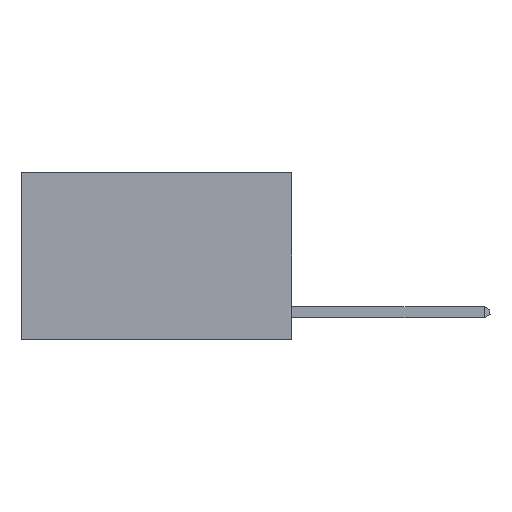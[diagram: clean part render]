
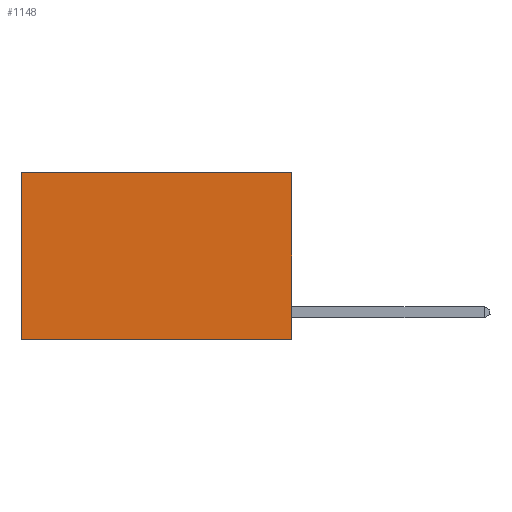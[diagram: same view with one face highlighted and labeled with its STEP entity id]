
A CAD part, left-side view. The second image highlights one B-rep face of the part: STEP entity #1148.
In plain terms, the highlighted planar face has unit normal (-1, 0, 0).
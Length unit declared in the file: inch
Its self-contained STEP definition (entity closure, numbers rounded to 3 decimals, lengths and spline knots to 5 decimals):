
#191 = VECTOR ( 'NONE', #1075, 39.37008 ) ;
#403 = CARTESIAN_POINT ( 'NONE',  ( 0.2625, 0., 0. ) ) ;
#1075 = DIRECTION ( 'NONE',  ( 0., 0., -1. ) ) ;
#1078 = VECTOR ( 'NONE', #3382, 39.37008 ) ;
#1148 = ADVANCED_FACE ( 'NONE', ( #2878 ), #8257, .F. ) ;
#1257 = AXIS2_PLACEMENT_3D ( 'NONE', #2298, #6361, #3624 ) ;
#1353 = VECTOR ( 'NONE', #2672, 39.37008 ) ;
#1449 = EDGE_LOOP ( 'NONE', ( #6391, #7226, #7127, #5285 ) ) ;
#1949 = EDGE_CURVE ( 'NONE', #7722, #6297, #4508, .T. ) ;
#2012 = CARTESIAN_POINT ( 'NONE',  ( 0.2625, 0.6, 0. ) ) ;
#2298 = CARTESIAN_POINT ( 'NONE',  ( 0.2625, 0., 0. ) ) ;
#2380 = CARTESIAN_POINT ( 'NONE',  ( 0.2625, 0., 0. ) ) ;
#2588 = CARTESIAN_POINT ( 'NONE',  ( 0.2625, 0., -0.37 ) ) ;
#2672 = DIRECTION ( 'NONE',  ( 0., 1., 0. ) ) ;
#2878 = FACE_OUTER_BOUND ( 'NONE', #1449, .T. ) ;
#2935 = CARTESIAN_POINT ( 'NONE',  ( 0.2625, 0.6, -0.37 ) ) ;
#3247 = LINE ( 'NONE', #2380, #191 ) ;
#3382 = DIRECTION ( 'NONE',  ( 0., 0., -1. ) ) ;
#3442 = VERTEX_POINT ( 'NONE', #7729 ) ;
#3558 = EDGE_CURVE ( 'NONE', #3442, #4061, #4489, .T. ) ;
#3624 = DIRECTION ( 'NONE',  ( 0., 0., -1. ) ) ;
#4061 = VERTEX_POINT ( 'NONE', #2935 ) ;
#4489 = LINE ( 'NONE', #2588, #1353 ) ;
#4508 = LINE ( 'NONE', #8424, #8647 ) ;
#5285 = ORIENTED_EDGE ( 'NONE', *, *, #1949, .T. ) ;
#6267 = EDGE_CURVE ( 'NONE', #7722, #3442, #3247, .T. ) ;
#6297 = VERTEX_POINT ( 'NONE', #8079 ) ;
#6361 = DIRECTION ( 'NONE',  ( 1., 0., 0. ) ) ;
#6391 = ORIENTED_EDGE ( 'NONE', *, *, #6738, .T. ) ;
#6554 = LINE ( 'NONE', #2012, #1078 ) ;
#6738 = EDGE_CURVE ( 'NONE', #6297, #4061, #6554, .T. ) ;
#7127 = ORIENTED_EDGE ( 'NONE', *, *, #6267, .F. ) ;
#7226 = ORIENTED_EDGE ( 'NONE', *, *, #3558, .F. ) ;
#7722 = VERTEX_POINT ( 'NONE', #403 ) ;
#7729 = CARTESIAN_POINT ( 'NONE',  ( 0.2625, 0., -0.37 ) ) ;
#7848 = DIRECTION ( 'NONE',  ( 0., 1., 0. ) ) ;
#8079 = CARTESIAN_POINT ( 'NONE',  ( 0.2625, 0.6, 0. ) ) ;
#8257 = PLANE ( 'NONE',  #1257 ) ;
#8424 = CARTESIAN_POINT ( 'NONE',  ( 0.2625, 0., 0. ) ) ;
#8647 = VECTOR ( 'NONE', #7848, 39.37008 ) ;
